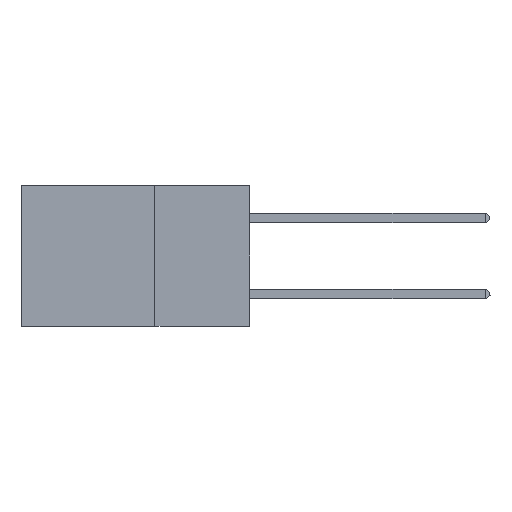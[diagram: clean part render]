
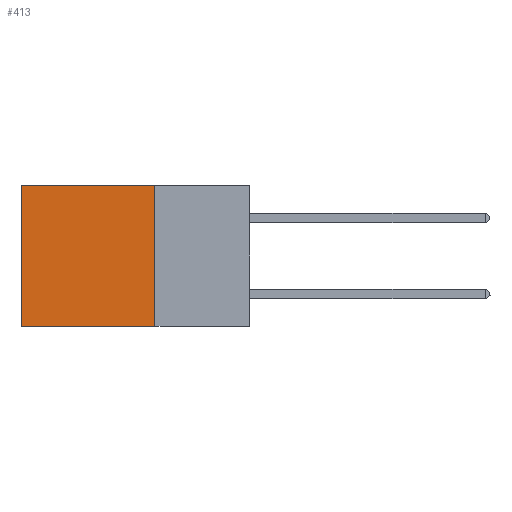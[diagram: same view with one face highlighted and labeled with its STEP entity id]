
A CAD part, left-side view. The second image highlights one B-rep face of the part: STEP entity #413.
In plain terms, the highlighted planar face has unit normal (-1, 0, 0).
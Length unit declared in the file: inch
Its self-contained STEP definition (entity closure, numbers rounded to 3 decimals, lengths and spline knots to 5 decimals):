
#42 = CARTESIAN_POINT ( 'NONE',  ( 0.2875, 0.25, 0. ) ) ;
#413 = ADVANCED_FACE ( 'NONE', ( #3254 ), #18560, .F. ) ;
#1383 = CARTESIAN_POINT ( 'NONE',  ( 0.2875, 0.25, 0. ) ) ;
#3254 = FACE_OUTER_BOUND ( 'NONE', #36215, .T. ) ;
#3311 = DIRECTION ( 'NONE',  ( 0., 0., -1. ) ) ;
#5303 = CARTESIAN_POINT ( 'NONE',  ( 0.2875, 0.25, -0.37 ) ) ;
#5512 = LINE ( 'NONE', #28747, #19849 ) ;
#6568 = DIRECTION ( 'NONE',  ( 0., 1., 0. ) ) ;
#6781 = CARTESIAN_POINT ( 'NONE',  ( 0.2875, 0.6, -0.37 ) ) ;
#9076 = DIRECTION ( 'NONE',  ( 0., 0., -1. ) ) ;
#9642 = LINE ( 'NONE', #42, #38803 ) ;
#10470 = VECTOR ( 'NONE', #6568, 39.37008 ) ;
#12963 = EDGE_CURVE ( 'NONE', #28381, #35144, #5512, .T. ) ;
#14817 = ORIENTED_EDGE ( 'NONE', *, *, #39520, .F. ) ;
#18169 = EDGE_CURVE ( 'NONE', #34477, #35144, #38868, .T. ) ;
#18560 = PLANE ( 'NONE',  #35778 ) ;
#19849 = VECTOR ( 'NONE', #34602, 39.37008 ) ;
#21921 = EDGE_CURVE ( 'NONE', #32423, #28381, #24718, .T. ) ;
#21973 = CARTESIAN_POINT ( 'NONE',  ( 0.2875, 0.25, 0. ) ) ;
#24718 = LINE ( 'NONE', #28748, #10470 ) ;
#24856 = DIRECTION ( 'NONE',  ( 1., 0., 0. ) ) ;
#28381 = VERTEX_POINT ( 'NONE', #33248 ) ;
#28747 = CARTESIAN_POINT ( 'NONE',  ( 0.2875, 0.6, 0. ) ) ;
#28748 = CARTESIAN_POINT ( 'NONE',  ( 0.2875, 0.25, 0. ) ) ;
#31553 = ORIENTED_EDGE ( 'NONE', *, *, #21921, .T. ) ;
#32423 = VERTEX_POINT ( 'NONE', #1383 ) ;
#33248 = CARTESIAN_POINT ( 'NONE',  ( 0.2875, 0.6, 0. ) ) ;
#34477 = VERTEX_POINT ( 'NONE', #38435 ) ;
#34602 = DIRECTION ( 'NONE',  ( 0., 0., -1. ) ) ;
#35144 = VERTEX_POINT ( 'NONE', #6781 ) ;
#35778 = AXIS2_PLACEMENT_3D ( 'NONE', #21973, #24856, #3311 ) ;
#36215 = EDGE_LOOP ( 'NONE', ( #40034, #39760, #14817, #31553 ) ) ;
#37855 = VECTOR ( 'NONE', #40213, 39.37008 ) ;
#38435 = CARTESIAN_POINT ( 'NONE',  ( 0.2875, 0.25, -0.37 ) ) ;
#38803 = VECTOR ( 'NONE', #9076, 39.37008 ) ;
#38868 = LINE ( 'NONE', #5303, #37855 ) ;
#39520 = EDGE_CURVE ( 'NONE', #32423, #34477, #9642, .T. ) ;
#39760 = ORIENTED_EDGE ( 'NONE', *, *, #18169, .F. ) ;
#40034 = ORIENTED_EDGE ( 'NONE', *, *, #12963, .T. ) ;
#40213 = DIRECTION ( 'NONE',  ( 0., 1., 0. ) ) ;
